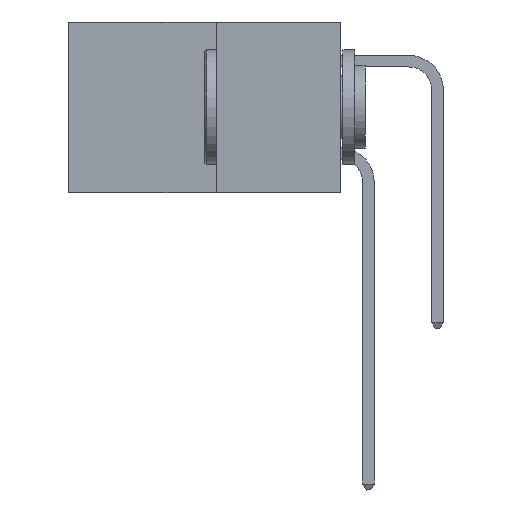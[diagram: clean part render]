
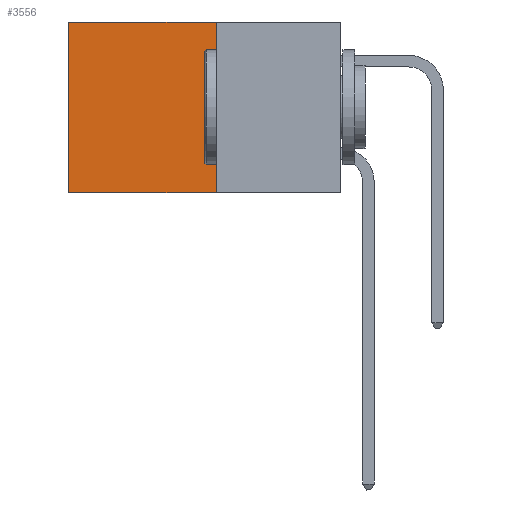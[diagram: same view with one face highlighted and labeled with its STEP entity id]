
A CAD part, left-side view. The second image highlights one B-rep face of the part: STEP entity #3556.
In plain terms, the highlighted planar face has unit normal (-1, 0, 0).
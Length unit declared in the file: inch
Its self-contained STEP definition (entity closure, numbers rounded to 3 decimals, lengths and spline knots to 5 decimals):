
#201 = CARTESIAN_POINT ( 'NONE',  ( 0.277, 0.27, -0.37 ) ) ;
#314 = CARTESIAN_POINT ( 'NONE',  ( 0.277, 0.27, 0. ) ) ;
#378 = DIRECTION ( 'NONE',  ( 0., 1., 0. ) ) ;
#506 = EDGE_CURVE ( 'NONE', #1565, #3069, #14209, .T. ) ;
#909 = CARTESIAN_POINT ( 'NONE',  ( 0.277, 0.27, -0.37 ) ) ;
#1285 = AXIS2_PLACEMENT_3D ( 'NONE', #10656, #9057, #16787 ) ;
#1565 = VERTEX_POINT ( 'NONE', #2882 ) ;
#1657 = DIRECTION ( 'NONE',  ( 0., 0., -1. ) ) ;
#2078 = LINE ( 'NONE', #201, #9130 ) ;
#2882 = CARTESIAN_POINT ( 'NONE',  ( 0.277, 0.59, 0. ) ) ;
#3069 = VERTEX_POINT ( 'NONE', #9007 ) ;
#3414 = LINE ( 'NONE', #3572, #13692 ) ;
#3556 = ADVANCED_FACE ( 'NONE', ( #13893 ), #8311, .F. ) ;
#3572 = CARTESIAN_POINT ( 'NONE',  ( 0.277, 0.27, -0.37 ) ) ;
#3596 = DIRECTION ( 'NONE',  ( 0., 1., 0. ) ) ;
#3950 = ORIENTED_EDGE ( 'NONE', *, *, #506, .T. ) ;
#5277 = EDGE_CURVE ( 'NONE', #5410, #1565, #8170, .T. ) ;
#5410 = VERTEX_POINT ( 'NONE', #17164 ) ;
#6197 = DIRECTION ( 'NONE',  ( 0., 0., -1. ) ) ;
#6630 = ORIENTED_EDGE ( 'NONE', *, *, #9497, .F. ) ;
#8170 = LINE ( 'NONE', #314, #14245 ) ;
#8311 = PLANE ( 'NONE',  #1285 ) ;
#9007 = CARTESIAN_POINT ( 'NONE',  ( 0.277, 0.59, -0.37 ) ) ;
#9057 = DIRECTION ( 'NONE',  ( 1., 0., 0. ) ) ;
#9130 = VECTOR ( 'NONE', #1657, 39.37008 ) ;
#9497 = EDGE_CURVE ( 'NONE', #11184, #3069, #3414, .T. ) ;
#10515 = VECTOR ( 'NONE', #6197, 39.37008 ) ;
#10656 = CARTESIAN_POINT ( 'NONE',  ( 0.277, 0.27, -0.37 ) ) ;
#10980 = ORIENTED_EDGE ( 'NONE', *, *, #18024, .F. ) ;
#11184 = VERTEX_POINT ( 'NONE', #909 ) ;
#11204 = CARTESIAN_POINT ( 'NONE',  ( 0.277, 0.59, -0.37 ) ) ;
#13692 = VECTOR ( 'NONE', #3596, 39.37008 ) ;
#13893 = FACE_OUTER_BOUND ( 'NONE', #17262, .T. ) ;
#14209 = LINE ( 'NONE', #11204, #10515 ) ;
#14245 = VECTOR ( 'NONE', #378, 39.37008 ) ;
#16787 = DIRECTION ( 'NONE',  ( 0., 0., -1. ) ) ;
#16815 = ORIENTED_EDGE ( 'NONE', *, *, #5277, .T. ) ;
#17164 = CARTESIAN_POINT ( 'NONE',  ( 0.277, 0.27, 0. ) ) ;
#17262 = EDGE_LOOP ( 'NONE', ( #3950, #6630, #10980, #16815 ) ) ;
#18024 = EDGE_CURVE ( 'NONE', #5410, #11184, #2078, .T. ) ;
